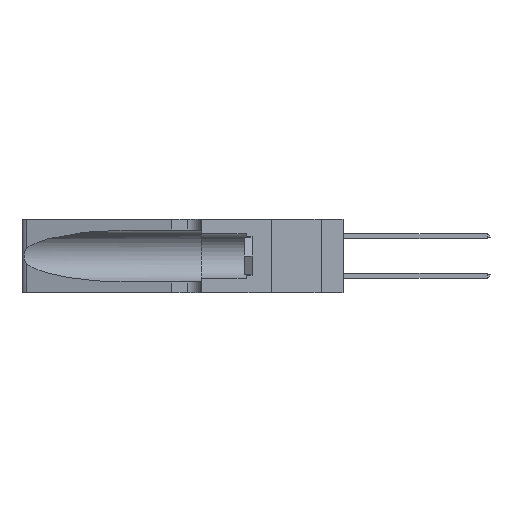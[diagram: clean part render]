
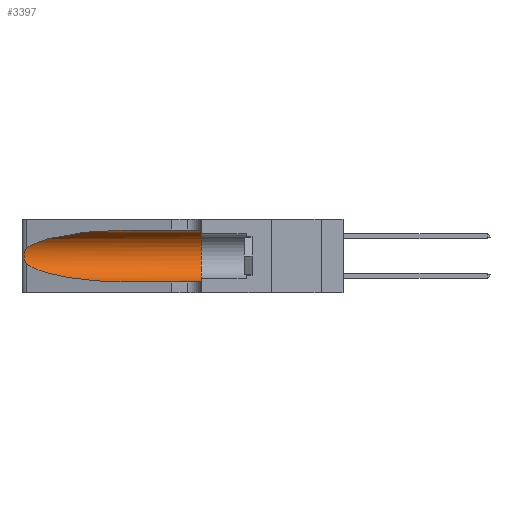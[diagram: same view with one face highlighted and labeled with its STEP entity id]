
A CAD part, left-side view. The second image highlights one B-rep face of the part: STEP entity #3397.
In plain terms, the highlighted cylindrical face has radius 3.308 mm (diameter 6.617 mm), a partial arc.
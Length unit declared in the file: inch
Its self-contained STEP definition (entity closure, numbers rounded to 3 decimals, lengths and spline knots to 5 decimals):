
#264 = B_SPLINE_CURVE_WITH_KNOTS ( 'NONE', 3,
 ( #23938, #9203, #13488, #654, #15631, #2859, #17776, #5002, #19860, #7173, #21927, #9294, #24023, #11475 ),
 .UNSPECIFIED., .F., .F.,
 ( 4, 2, 2, 2, 2, 2, 4 ),
 ( 0., 0.00027, 0.00053, 0.00107, 0.0016, 0.00187, 0.00214 ),
 .UNSPECIFIED. ) ;
#654 = CARTESIAN_POINT ( 'NONE',  ( 0.25787, 1.23484, 0.2124 ) ) ;
#1385 = FACE_OUTER_BOUND ( 'NONE', #10479, .T. ) ;
#1888 = CARTESIAN_POINT ( 'NONE',  ( 0.25487, 1.22718, 0.14631 ) ) ;
#1967 = ORIENTED_EDGE ( 'NONE', *, *, #17778, .T. ) ;
#2859 = CARTESIAN_POINT ( 'NONE',  ( 0.26018, 1.23835, 0.19895 ) ) ;
#3380 = LINE ( 'NONE', #24510, #14046 ) ;
#3397 = ADVANCED_FACE ( 'NONE', ( #1385 ), #12120, .F. ) ;
#3791 = ORIENTED_EDGE ( 'NONE', *, *, #15843, .F. ) ;
#4441 = CARTESIAN_POINT ( 'NONE',  ( 0.2373, 1.15595, 0.08982 ) ) ;
#5002 = CARTESIAN_POINT ( 'NONE',  ( 0.26075, 1.23896, 0.178 ) ) ;
#5175 = ORIENTED_EDGE ( 'NONE', *, *, #11813, .F. ) ;
#5591 = DIRECTION ( 'NONE',  ( 0., -1., 0. ) ) ;
#6607 = CARTESIAN_POINT ( 'NONE',  ( 0.1305, 0.72297, 0.05475 ) ) ;
#6668 = LINE ( 'NONE', #7908, #22181 ) ;
#6977 = VERTEX_POINT ( 'NONE', #14912 ) ;
#7173 = CARTESIAN_POINT ( 'NONE',  ( 0.25856, 1.23593, 0.16098 ) ) ;
#7789 = ORIENTED_EDGE ( 'NONE', *, *, #20545, .T. ) ;
#7908 = CARTESIAN_POINT ( 'NONE',  ( 0.1305, 1.61858, 0.31525 ) ) ;
#8034 = CARTESIAN_POINT ( 'NONE',  ( 0.18966, 0.96281, 0.31525 ) ) ;
#8368 = DIRECTION ( 'NONE',  ( 0., 1., 0. ) ) ;
#8640 = AXIS2_PLACEMENT_3D ( 'NONE', #25509, #15087, #21316 ) ;
#9203 = CARTESIAN_POINT ( 'NONE',  ( 0.25555, 1.22994, 0.2215 ) ) ;
#9294 = CARTESIAN_POINT ( 'NONE',  ( 0.25639, 1.23186, 0.15144 ) ) ;
#9632 = VERTEX_POINT ( 'NONE', #1888 ) ;
#9932 =( BOUNDED_CURVE ( )  B_SPLINE_CURVE ( 3, ( #22781, #8034, #12330, #27005 ),
 .UNSPECIFIED., .F., .T. ) 
 B_SPLINE_CURVE_WITH_KNOTS ( ( 4, 4 ),
 ( 1.5708, 2.84003 ),
 .UNSPECIFIED. ) 
 CURVE ( )  GEOMETRIC_REPRESENTATION_ITEM ( )  RATIONAL_B_SPLINE_CURVE ( ( 1., 0.87, 0.87, 1. ) ) 
 REPRESENTATION_ITEM ( '' )  );
#10479 = EDGE_LOOP ( 'NONE', ( #22902, #1967, #7789, #12931, #3791, #5175 ) ) ;
#11475 = CARTESIAN_POINT ( 'NONE',  ( 0.25487, 1.22718, 0.14631 ) ) ;
#11813 = EDGE_CURVE ( 'NONE', #6977, #16883, #6668, .T. ) ;
#12120 = CYLINDRICAL_SURFACE ( 'NONE', #8640, 0.13025 ) ;
#12330 = CARTESIAN_POINT ( 'NONE',  ( 0.2373, 1.15595, 0.28018 ) ) ;
#12931 = ORIENTED_EDGE ( 'NONE', *, *, #14980, .T. ) ;
#13488 = CARTESIAN_POINT ( 'NONE',  ( 0.25639, 1.23184, 0.21858 ) ) ;
#14046 = VECTOR ( 'NONE', #5591, 39.37008 ) ;
#14136 = VERTEX_POINT ( 'NONE', #26295 ) ;
#14194 = AXIS2_PLACEMENT_3D ( 'NONE', #21021, #8368, #23113 ) ;
#14875 =( BOUNDED_CURVE ( )  B_SPLINE_CURVE ( 3, ( #17214, #4441, #19324, #6607 ),
 .UNSPECIFIED., .F., .F. ) 
 B_SPLINE_CURVE_WITH_KNOTS ( ( 4, 4 ),
 ( 3.44316, 4.71239 ),
 .UNSPECIFIED. ) 
 CURVE ( )  GEOMETRIC_REPRESENTATION_ITEM ( )  RATIONAL_B_SPLINE_CURVE ( ( 1., 0.87, 0.87, 1. ) ) 
 REPRESENTATION_ITEM ( '' )  );
#14912 = CARTESIAN_POINT ( 'NONE',  ( 0.1305, 0.72297, 0.31525 ) ) ;
#14980 = EDGE_CURVE ( 'NONE', #27373, #22928, #3380, .T. ) ;
#15087 = DIRECTION ( 'NONE',  ( 0., -1., 0. ) ) ;
#15333 = CIRCLE ( 'NONE', #14194, 0.13025 ) ;
#15631 = CARTESIAN_POINT ( 'NONE',  ( 0.25854, 1.2359, 0.20912 ) ) ;
#15843 = EDGE_CURVE ( 'NONE', #16883, #22928, #15333, .T. ) ;
#16883 = VERTEX_POINT ( 'NONE', #17083 ) ;
#17083 = CARTESIAN_POINT ( 'NONE',  ( 0.1305, 0.35, 0.31525 ) ) ;
#17214 = CARTESIAN_POINT ( 'NONE',  ( 0.25487, 1.22718, 0.14631 ) ) ;
#17776 = CARTESIAN_POINT ( 'NONE',  ( 0.26075, 1.23896, 0.19203 ) ) ;
#17778 = EDGE_CURVE ( 'NONE', #14136, #9632, #264, .T. ) ;
#18212 = CARTESIAN_POINT ( 'NONE',  ( 0.1305, 0.72297, 0.05475 ) ) ;
#19261 = EDGE_CURVE ( 'NONE', #6977, #14136, #9932, .T. ) ;
#19324 = CARTESIAN_POINT ( 'NONE',  ( 0.18966, 0.96281, 0.05475 ) ) ;
#19860 = CARTESIAN_POINT ( 'NONE',  ( 0.26017, 1.23833, 0.17102 ) ) ;
#20545 = EDGE_CURVE ( 'NONE', #9632, #27373, #14875, .T. ) ;
#20885 = CARTESIAN_POINT ( 'NONE',  ( 0.1305, 0.35, 0.05475 ) ) ;
#21021 = CARTESIAN_POINT ( 'NONE',  ( 0.1305, 0.35, 0.185 ) ) ;
#21316 = DIRECTION ( 'NONE',  ( 0., 0., -1. ) ) ;
#21927 = CARTESIAN_POINT ( 'NONE',  ( 0.25789, 1.23486, 0.15765 ) ) ;
#22181 = VECTOR ( 'NONE', #26885, 39.37008 ) ;
#22781 = CARTESIAN_POINT ( 'NONE',  ( 0.1305, 0.72297, 0.31525 ) ) ;
#22902 = ORIENTED_EDGE ( 'NONE', *, *, #19261, .T. ) ;
#22928 = VERTEX_POINT ( 'NONE', #20885 ) ;
#23113 = DIRECTION ( 'NONE',  ( 0., 0., 1. ) ) ;
#23938 = CARTESIAN_POINT ( 'NONE',  ( 0.25487, 1.22718, 0.22369 ) ) ;
#24023 = CARTESIAN_POINT ( 'NONE',  ( 0.25555, 1.22993, 0.14849 ) ) ;
#24510 = CARTESIAN_POINT ( 'NONE',  ( 0.1305, 1.61858, 0.05475 ) ) ;
#25509 = CARTESIAN_POINT ( 'NONE',  ( 0.1305, 1.61858, 0.185 ) ) ;
#26295 = CARTESIAN_POINT ( 'NONE',  ( 0.25487, 1.22718, 0.22369 ) ) ;
#26885 = DIRECTION ( 'NONE',  ( 0., -1., 0. ) ) ;
#27005 = CARTESIAN_POINT ( 'NONE',  ( 0.25487, 1.22718, 0.22369 ) ) ;
#27373 = VERTEX_POINT ( 'NONE', #18212 ) ;
